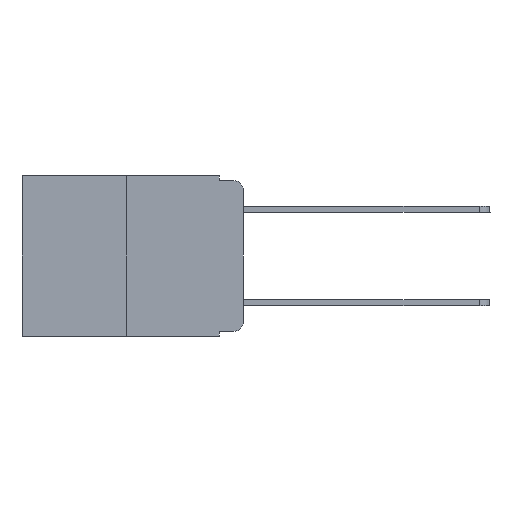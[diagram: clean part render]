
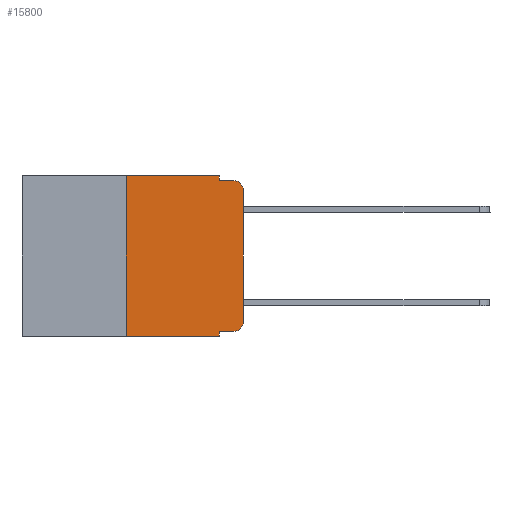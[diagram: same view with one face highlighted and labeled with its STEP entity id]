
A CAD part, left-side view. The second image highlights one B-rep face of the part: STEP entity #15800.
In plain terms, the highlighted planar face has unit normal (-1, 0, 0).
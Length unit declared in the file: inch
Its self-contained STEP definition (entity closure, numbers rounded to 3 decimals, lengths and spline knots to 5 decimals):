
#241 = LINE ( 'NONE', #20941, #4345 ) ;
#325 = VERTEX_POINT ( 'NONE', #18810 ) ;
#485 = LINE ( 'NONE', #4951, #22491 ) ;
#533 = LINE ( 'NONE', #17735, #21059 ) ;
#857 = LINE ( 'NONE', #8513, #10768 ) ;
#1060 = CARTESIAN_POINT ( 'NONE',  ( 0., 0.051, 0. ) ) ;
#1145 = DIRECTION ( 'NONE',  ( 0., 0., -1. ) ) ;
#1391 = CARTESIAN_POINT ( 'NONE',  ( 0., 0.02, -0.333 ) ) ;
#1496 = EDGE_CURVE ( 'NONE', #13853, #1779, #485, .T. ) ;
#1779 = VERTEX_POINT ( 'NONE', #5848 ) ;
#1989 = LINE ( 'NONE', #21913, #13091 ) ;
#1994 = CIRCLE ( 'NONE', #10782, 0.02 ) ;
#2024 = DIRECTION ( 'NONE',  ( 0., 0., 1. ) ) ;
#3058 = VERTEX_POINT ( 'NONE', #13534 ) ;
#3142 = CARTESIAN_POINT ( 'NONE',  ( 0., 0.473, 0. ) ) ;
#4027 = CARTESIAN_POINT ( 'NONE',  ( 0., 0.051, 0. ) ) ;
#4130 = ORIENTED_EDGE ( 'NONE', *, *, #18666, .T. ) ;
#4345 = VECTOR ( 'NONE', #2024, 39.37008 ) ;
#4532 = DIRECTION ( 'NONE',  ( 0., 0., -1. ) ) ;
#4605 = EDGE_LOOP ( 'NONE', ( #15821, #18411, #9192, #19490, #21525, #23413, #16555, #21719, #4130, #5963 ) ) ;
#4746 = EDGE_CURVE ( 'NONE', #325, #1779, #5921, .T. ) ;
#4951 = CARTESIAN_POINT ( 'NONE',  ( 0., 0.051, -0.01 ) ) ;
#5152 = AXIS2_PLACEMENT_3D ( 'NONE', #17753, #23190, #11902 ) ;
#5162 = EDGE_CURVE ( 'NONE', #22056, #13853, #19394, .T. ) ;
#5848 = CARTESIAN_POINT ( 'NONE',  ( 0., 0.02, -0.01 ) ) ;
#5921 = CIRCLE ( 'NONE', #5152, 0.02 ) ;
#5963 = ORIENTED_EDGE ( 'NONE', *, *, #18560, .T. ) ;
#6271 = CARTESIAN_POINT ( 'NONE',  ( 0., 0.02, -0.313 ) ) ;
#7928 = AXIS2_PLACEMENT_3D ( 'NONE', #19876, #14261, #19719 ) ;
#7934 = LINE ( 'NONE', #3142, #18517 ) ;
#8019 = EDGE_CURVE ( 'NONE', #10432, #325, #241, .T. ) ;
#8472 = EDGE_CURVE ( 'NONE', #3058, #10019, #1989, .T. ) ;
#8513 = CARTESIAN_POINT ( 'NONE',  ( 0., 0.25, 0. ) ) ;
#9192 = ORIENTED_EDGE ( 'NONE', *, *, #1496, .F. ) ;
#10019 = VERTEX_POINT ( 'NONE', #16368 ) ;
#10432 = VERTEX_POINT ( 'NONE', #17439 ) ;
#10630 = LINE ( 'NONE', #19514, #21519 ) ;
#10768 = VECTOR ( 'NONE', #17786, 39.37008 ) ;
#10782 = AXIS2_PLACEMENT_3D ( 'NONE', #6271, #13929, #4532 ) ;
#10810 = DIRECTION ( 'NONE',  ( 0., -1., 0. ) ) ;
#10879 = EDGE_CURVE ( 'NONE', #15342, #10019, #10630, .T. ) ;
#11902 = DIRECTION ( 'NONE',  ( 0., 0., -1. ) ) ;
#12449 = DIRECTION ( 'NONE',  ( 0., -1., 0. ) ) ;
#13091 = VECTOR ( 'NONE', #10810, 39.37008 ) ;
#13193 = VECTOR ( 'NONE', #1145, 39.37008 ) ;
#13485 = FACE_OUTER_BOUND ( 'NONE', #4605, .T. ) ;
#13534 = CARTESIAN_POINT ( 'NONE',  ( 0., 0.25, -0.343 ) ) ;
#13725 = VERTEX_POINT ( 'NONE', #21165 ) ;
#13853 = VERTEX_POINT ( 'NONE', #17024 ) ;
#13929 = DIRECTION ( 'NONE',  ( -1., 0., 0. ) ) ;
#14261 = DIRECTION ( 'NONE',  ( 1., 0., 0. ) ) ;
#15342 = VERTEX_POINT ( 'NONE', #16345 ) ;
#15765 = EDGE_CURVE ( 'NONE', #13725, #22056, #7934, .T. ) ;
#15800 = ADVANCED_FACE ( 'NONE', ( #13485 ), #19802, .F. ) ;
#15821 = ORIENTED_EDGE ( 'NONE', *, *, #8019, .T. ) ;
#16345 = CARTESIAN_POINT ( 'NONE',  ( 0., 0.051, -0.333 ) ) ;
#16368 = CARTESIAN_POINT ( 'NONE',  ( 0., 0.051, -0.343 ) ) ;
#16555 = ORIENTED_EDGE ( 'NONE', *, *, #8472, .T. ) ;
#17024 = CARTESIAN_POINT ( 'NONE',  ( 0., 0.051, -0.01 ) ) ;
#17439 = CARTESIAN_POINT ( 'NONE',  ( 0., 0., -0.313 ) ) ;
#17708 = DIRECTION ( 'NONE',  ( 0., 0., -1. ) ) ;
#17735 = CARTESIAN_POINT ( 'NONE',  ( 0., 0.051, -0.333 ) ) ;
#17753 = CARTESIAN_POINT ( 'NONE',  ( 0., 0.02, -0.03 ) ) ;
#17786 = DIRECTION ( 'NONE',  ( 0., 0., 1. ) ) ;
#18411 = ORIENTED_EDGE ( 'NONE', *, *, #4746, .T. ) ;
#18517 = VECTOR ( 'NONE', #21609, 39.37008 ) ;
#18560 = EDGE_CURVE ( 'NONE', #19283, #10432, #1994, .T. ) ;
#18666 = EDGE_CURVE ( 'NONE', #15342, #19283, #533, .T. ) ;
#18810 = CARTESIAN_POINT ( 'NONE',  ( 0., 0., -0.03 ) ) ;
#19283 = VERTEX_POINT ( 'NONE', #1391 ) ;
#19394 = LINE ( 'NONE', #1060, #13193 ) ;
#19490 = ORIENTED_EDGE ( 'NONE', *, *, #5162, .F. ) ;
#19514 = CARTESIAN_POINT ( 'NONE',  ( 0., 0.051, 0. ) ) ;
#19719 = DIRECTION ( 'NONE',  ( 0., 0., -1. ) ) ;
#19802 = PLANE ( 'NONE',  #7928 ) ;
#19876 = CARTESIAN_POINT ( 'NONE',  ( 0., 0.473, 0. ) ) ;
#20941 = CARTESIAN_POINT ( 'NONE',  ( 0., 0., 0. ) ) ;
#21059 = VECTOR ( 'NONE', #12449, 39.37008 ) ;
#21165 = CARTESIAN_POINT ( 'NONE',  ( 0., 0.25, 0. ) ) ;
#21519 = VECTOR ( 'NONE', #17708, 39.37008 ) ;
#21525 = ORIENTED_EDGE ( 'NONE', *, *, #15765, .F. ) ;
#21609 = DIRECTION ( 'NONE',  ( 0., -1., 0. ) ) ;
#21719 = ORIENTED_EDGE ( 'NONE', *, *, #10879, .F. ) ;
#21913 = CARTESIAN_POINT ( 'NONE',  ( 0., 0.473, -0.343 ) ) ;
#22056 = VERTEX_POINT ( 'NONE', #4027 ) ;
#22087 = DIRECTION ( 'NONE',  ( 0., -1., 0. ) ) ;
#22305 = EDGE_CURVE ( 'NONE', #3058, #13725, #857, .T. ) ;
#22491 = VECTOR ( 'NONE', #22087, 39.37008 ) ;
#23190 = DIRECTION ( 'NONE',  ( -1., 0., 0. ) ) ;
#23413 = ORIENTED_EDGE ( 'NONE', *, *, #22305, .F. ) ;
